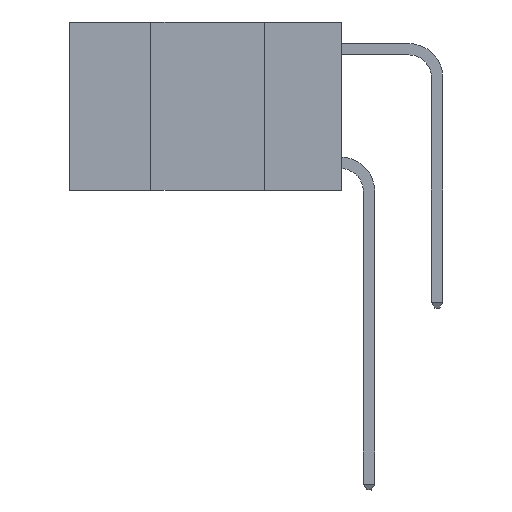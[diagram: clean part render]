
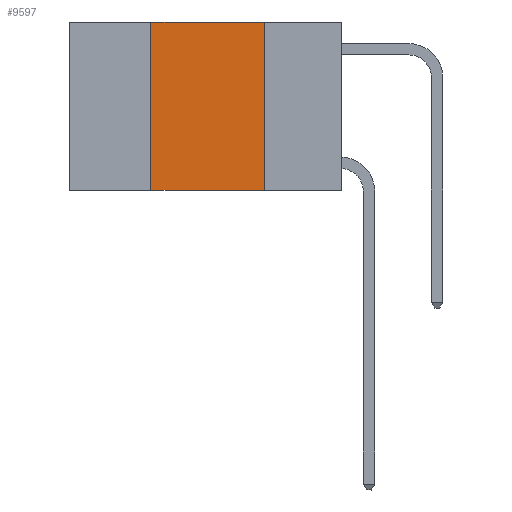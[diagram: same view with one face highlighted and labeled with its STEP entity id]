
A CAD part, left-side view. The second image highlights one B-rep face of the part: STEP entity #9597.
In plain terms, the highlighted planar face has unit normal (-1, 0, 0).
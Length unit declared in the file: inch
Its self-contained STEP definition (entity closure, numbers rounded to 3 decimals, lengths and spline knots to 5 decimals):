
#602 = CARTESIAN_POINT ( 'NONE',  ( 0., 0.17, 0. ) ) ;
#1366 = EDGE_LOOP ( 'NONE', ( #3942, #19578, #21216, #4853 ) ) ;
#2376 = CARTESIAN_POINT ( 'NONE',  ( 0., 0.42, 0. ) ) ;
#3942 = ORIENTED_EDGE ( 'NONE', *, *, #20001, .F. ) ;
#4299 = EDGE_CURVE ( 'NONE', #19397, #7573, #23406, .T. ) ;
#4707 = CARTESIAN_POINT ( 'NONE',  ( 0., 0.6, 0. ) ) ;
#4810 = LINE ( 'NONE', #602, #7906 ) ;
#4853 = ORIENTED_EDGE ( 'NONE', *, *, #22857, .T. ) ;
#4862 = LINE ( 'NONE', #13015, #8319 ) ;
#5059 = DIRECTION ( 'NONE',  ( 0., 0., -1. ) ) ;
#6974 = EDGE_CURVE ( 'NONE', #7573, #9366, #10079, .T. ) ;
#7573 = VERTEX_POINT ( 'NONE', #8451 ) ;
#7906 = VECTOR ( 'NONE', #5059, 39.37008 ) ;
#8050 = CARTESIAN_POINT ( 'NONE',  ( 0., 0.6, 0. ) ) ;
#8319 = VECTOR ( 'NONE', #10946, 39.37008 ) ;
#8451 = CARTESIAN_POINT ( 'NONE',  ( 0., 0.42, 0. ) ) ;
#9366 = VERTEX_POINT ( 'NONE', #20671 ) ;
#9597 = ADVANCED_FACE ( 'NONE', ( #23475 ), #14627, .F. ) ;
#10079 = LINE ( 'NONE', #8050, #22138 ) ;
#10946 = DIRECTION ( 'NONE',  ( 0., -1., 0. ) ) ;
#12983 = DIRECTION ( 'NONE',  ( 1., 0., 0. ) ) ;
#13015 = CARTESIAN_POINT ( 'NONE',  ( 0., 0.6, -0.37 ) ) ;
#13951 = CARTESIAN_POINT ( 'NONE',  ( 0., 0.17, -0.37 ) ) ;
#14500 = CARTESIAN_POINT ( 'NONE',  ( 0., 0.42, -0.37 ) ) ;
#14627 = PLANE ( 'NONE',  #15220 ) ;
#14834 = VERTEX_POINT ( 'NONE', #13951 ) ;
#15220 = AXIS2_PLACEMENT_3D ( 'NONE', #4707, #12983, #19251 ) ;
#19251 = DIRECTION ( 'NONE',  ( 0., 0., -1. ) ) ;
#19397 = VERTEX_POINT ( 'NONE', #14500 ) ;
#19578 = ORIENTED_EDGE ( 'NONE', *, *, #6974, .F. ) ;
#20001 = EDGE_CURVE ( 'NONE', #9366, #14834, #4810, .T. ) ;
#20671 = CARTESIAN_POINT ( 'NONE',  ( 0., 0.17, 0. ) ) ;
#21216 = ORIENTED_EDGE ( 'NONE', *, *, #4299, .F. ) ;
#22138 = VECTOR ( 'NONE', #24801, 39.37008 ) ;
#22565 = VECTOR ( 'NONE', #25565, 39.37008 ) ;
#22857 = EDGE_CURVE ( 'NONE', #19397, #14834, #4862, .T. ) ;
#23406 = LINE ( 'NONE', #2376, #22565 ) ;
#23475 = FACE_OUTER_BOUND ( 'NONE', #1366, .T. ) ;
#24801 = DIRECTION ( 'NONE',  ( 0., -1., 0. ) ) ;
#25565 = DIRECTION ( 'NONE',  ( 0., 0., 1. ) ) ;
